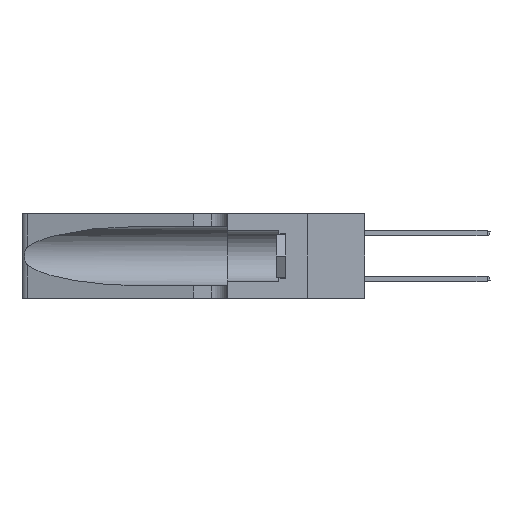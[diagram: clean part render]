
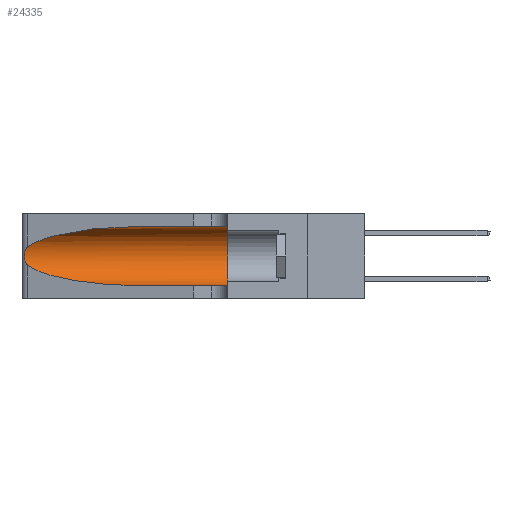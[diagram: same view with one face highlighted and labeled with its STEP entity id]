
A CAD part, left-side view. The second image highlights one B-rep face of the part: STEP entity #24335.
In plain terms, the highlighted cylindrical face has radius 3.308 mm (diameter 6.617 mm), a partial arc.
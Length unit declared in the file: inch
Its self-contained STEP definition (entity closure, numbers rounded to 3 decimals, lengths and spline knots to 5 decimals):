
#447 = CARTESIAN_POINT ( 'NONE',  ( 0.1305, 0.72297, 0.05475 ) ) ;
#1678 = ORIENTED_EDGE ( 'NONE', *, *, #25364, .T. ) ;
#1698 =( BOUNDED_CURVE ( )  B_SPLINE_CURVE ( 3, ( #19006, #25577, #23451, #10230 ),
 .UNSPECIFIED., .F., .T. ) 
 B_SPLINE_CURVE_WITH_KNOTS ( ( 4, 4 ),
 ( 3.44316, 4.71239 ),
 .UNSPECIFIED. ) 
 CURVE ( )  GEOMETRIC_REPRESENTATION_ITEM ( )  RATIONAL_B_SPLINE_CURVE ( ( 1., 0.87, 0.87, 1. ) ) 
 REPRESENTATION_ITEM ( '' )  );
#2033 = CARTESIAN_POINT ( 'NONE',  ( 0.26017, 1.23833, 0.17102 ) ) ;
#2338 = ORIENTED_EDGE ( 'NONE', *, *, #26536, .T. ) ;
#2340 = EDGE_LOOP ( 'NONE', ( #1678, #23791, #26460, #2338, #7562, #13865 ) ) ;
#3490 = CARTESIAN_POINT ( 'NONE',  ( 0.1305, 0.72297, 0.31525 ) ) ;
#3958 = FACE_OUTER_BOUND ( 'NONE', #2340, .T. ) ;
#4210 = VERTEX_POINT ( 'NONE', #20885 ) ;
#4290 = CARTESIAN_POINT ( 'NONE',  ( 0.25789, 1.23486, 0.15765 ) ) ;
#4641 = CARTESIAN_POINT ( 'NONE',  ( 0.2373, 1.15595, 0.28018 ) ) ;
#5056 = CARTESIAN_POINT ( 'NONE',  ( 0.25487, 1.22718, 0.14631 ) ) ;
#5805 = DIRECTION ( 'NONE',  ( 0., 1., 0. ) ) ;
#6328 = LINE ( 'NONE', #20053, #10784 ) ;
#6445 = CARTESIAN_POINT ( 'NONE',  ( 0.25639, 1.23184, 0.21858 ) ) ;
#6544 = CARTESIAN_POINT ( 'NONE',  ( 0.25555, 1.22993, 0.14849 ) ) ;
#7214 = CARTESIAN_POINT ( 'NONE',  ( 0.1305, 1.61858, 0.31525 ) ) ;
#7562 = ORIENTED_EDGE ( 'NONE', *, *, #15358, .F. ) ;
#8015 = AXIS2_PLACEMENT_3D ( 'NONE', #27965, #12513, #8090 ) ;
#8090 = DIRECTION ( 'NONE',  ( 0., 0., -1. ) ) ;
#8676 = CARTESIAN_POINT ( 'NONE',  ( 0.25487, 1.22718, 0.22369 ) ) ;
#9142 = EDGE_CURVE ( 'NONE', #11920, #9360, #12022, .T. ) ;
#9360 = VERTEX_POINT ( 'NONE', #5056 ) ;
#9387 = EDGE_CURVE ( 'NONE', #18225, #4210, #26559, .T. ) ;
#10230 = CARTESIAN_POINT ( 'NONE',  ( 0.1305, 0.72297, 0.05475 ) ) ;
#10784 = VECTOR ( 'NONE', #22265, 39.37008 ) ;
#10852 = CARTESIAN_POINT ( 'NONE',  ( 0.25787, 1.23484, 0.2124 ) ) ;
#11920 = VERTEX_POINT ( 'NONE', #16036 ) ;
#12022 = B_SPLINE_CURVE_WITH_KNOTS ( 'NONE', 3,
 ( #8676, #21874, #6445, #10852, #26318, #13087, #28516, #15300, #2033, #17529, #4290, #19753, #6544, #21968 ),
 .UNSPECIFIED., .F., .F.,
 ( 4, 2, 2, 2, 2, 2, 4 ),
 ( 0., 0.00027, 0.00053, 0.00107, 0.0016, 0.00187, 0.00214 ),
 .UNSPECIFIED. ) ;
#12513 = DIRECTION ( 'NONE',  ( 0., -1., 0. ) ) ;
#13087 = CARTESIAN_POINT ( 'NONE',  ( 0.26018, 1.23835, 0.19895 ) ) ;
#13787 = EDGE_CURVE ( 'NONE', #9360, #18664, #1698, .T. ) ;
#13865 = ORIENTED_EDGE ( 'NONE', *, *, #9387, .F. ) ;
#14216 = CIRCLE ( 'NONE', #23393, 0.13025 ) ;
#15034 = CYLINDRICAL_SURFACE ( 'NONE', #8015, 0.13025 ) ;
#15300 = CARTESIAN_POINT ( 'NONE',  ( 0.26075, 1.23896, 0.178 ) ) ;
#15358 = EDGE_CURVE ( 'NONE', #4210, #17277, #14216, .T. ) ;
#15657 = CARTESIAN_POINT ( 'NONE',  ( 0.18966, 0.96281, 0.31525 ) ) ;
#16036 = CARTESIAN_POINT ( 'NONE',  ( 0.25487, 1.22718, 0.22369 ) ) ;
#16166 = DIRECTION ( 'NONE',  ( 0., -1., 0. ) ) ;
#17277 = VERTEX_POINT ( 'NONE', #27616 ) ;
#17529 = CARTESIAN_POINT ( 'NONE',  ( 0.25856, 1.23593, 0.16098 ) ) ;
#17783 = CARTESIAN_POINT ( 'NONE',  ( 0.1305, 0.72297, 0.31525 ) ) ;
#18225 = VERTEX_POINT ( 'NONE', #3490 ) ;
#18664 = VERTEX_POINT ( 'NONE', #447 ) ;
#19006 = CARTESIAN_POINT ( 'NONE',  ( 0.25487, 1.22718, 0.14631 ) ) ;
#19011 = CARTESIAN_POINT ( 'NONE',  ( 0.1305, 0.35, 0.185 ) ) ;
#19753 = CARTESIAN_POINT ( 'NONE',  ( 0.25639, 1.23186, 0.15144 ) ) ;
#20053 = CARTESIAN_POINT ( 'NONE',  ( 0.1305, 1.61858, 0.05475 ) ) ;
#20106 = CARTESIAN_POINT ( 'NONE',  ( 0.25487, 1.22718, 0.22369 ) ) ;
#20697 = VECTOR ( 'NONE', #16166, 39.37008 ) ;
#20885 = CARTESIAN_POINT ( 'NONE',  ( 0.1305, 0.35, 0.31525 ) ) ;
#21253 = DIRECTION ( 'NONE',  ( 0., 0., 1. ) ) ;
#21874 = CARTESIAN_POINT ( 'NONE',  ( 0.25555, 1.22994, 0.2215 ) ) ;
#21968 = CARTESIAN_POINT ( 'NONE',  ( 0.25487, 1.22718, 0.14631 ) ) ;
#22265 = DIRECTION ( 'NONE',  ( 0., -1., 0. ) ) ;
#23393 = AXIS2_PLACEMENT_3D ( 'NONE', #19011, #5805, #21253 ) ;
#23451 = CARTESIAN_POINT ( 'NONE',  ( 0.18966, 0.96281, 0.05475 ) ) ;
#23791 = ORIENTED_EDGE ( 'NONE', *, *, #9142, .T. ) ;
#24335 = ADVANCED_FACE ( 'NONE', ( #3958 ), #15034, .F. ) ;
#25364 = EDGE_CURVE ( 'NONE', #18225, #11920, #28293, .T. ) ;
#25577 = CARTESIAN_POINT ( 'NONE',  ( 0.2373, 1.15595, 0.08982 ) ) ;
#26318 = CARTESIAN_POINT ( 'NONE',  ( 0.25854, 1.2359, 0.20912 ) ) ;
#26460 = ORIENTED_EDGE ( 'NONE', *, *, #13787, .T. ) ;
#26536 = EDGE_CURVE ( 'NONE', #18664, #17277, #6328, .T. ) ;
#26559 = LINE ( 'NONE', #7214, #20697 ) ;
#27616 = CARTESIAN_POINT ( 'NONE',  ( 0.1305, 0.35, 0.05475 ) ) ;
#27965 = CARTESIAN_POINT ( 'NONE',  ( 0.1305, 1.61858, 0.185 ) ) ;
#28293 =( BOUNDED_CURVE ( )  B_SPLINE_CURVE ( 3, ( #17783, #15657, #4641, #20106 ),
 .UNSPECIFIED., .F., .F. ) 
 B_SPLINE_CURVE_WITH_KNOTS ( ( 4, 4 ),
 ( 1.5708, 2.84003 ),
 .UNSPECIFIED. ) 
 CURVE ( )  GEOMETRIC_REPRESENTATION_ITEM ( )  RATIONAL_B_SPLINE_CURVE ( ( 1., 0.87, 0.87, 1. ) ) 
 REPRESENTATION_ITEM ( '' )  );
#28516 = CARTESIAN_POINT ( 'NONE',  ( 0.26075, 1.23896, 0.19203 ) ) ;
